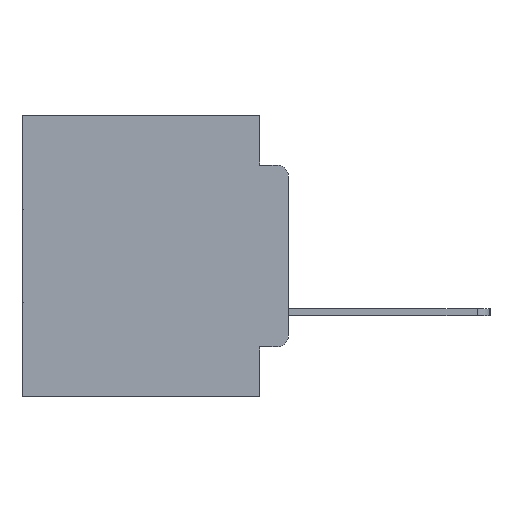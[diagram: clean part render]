
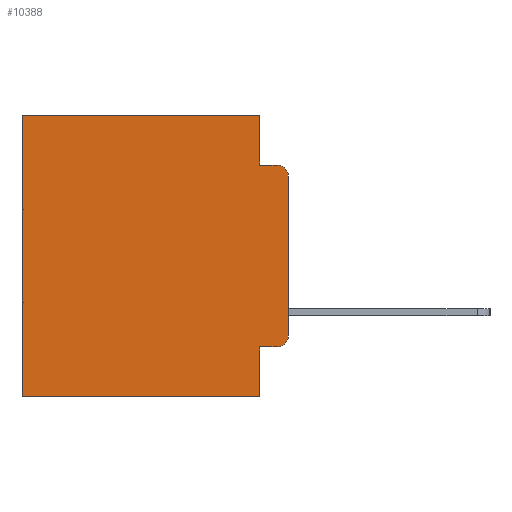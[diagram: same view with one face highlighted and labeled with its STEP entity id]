
A CAD part, left-side view. The second image highlights one B-rep face of the part: STEP entity #10388.
In plain terms, the highlighted planar face has unit normal (-1, 0, 0).
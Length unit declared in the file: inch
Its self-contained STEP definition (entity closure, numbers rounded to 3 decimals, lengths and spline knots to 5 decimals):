
#510 = ORIENTED_EDGE ( 'NONE', *, *, #28568, .F. ) ;
#564 = VECTOR ( 'NONE', #5904, 39.37008 ) ;
#1203 = ORIENTED_EDGE ( 'NONE', *, *, #3495, .T. ) ;
#1322 = AXIS2_PLACEMENT_3D ( 'NONE', #4643, #14088, #23806 ) ;
#1446 = CARTESIAN_POINT ( 'NONE',  ( 0.298, 0.02, -0.3915 ) ) ;
#1926 = DIRECTION ( 'NONE',  ( 0., 1., 0. ) ) ;
#1965 = LINE ( 'NONE', #17037, #8187 ) ;
#2395 = EDGE_CURVE ( 'NONE', #29765, #22675, #1965, .T. ) ;
#2718 = ORIENTED_EDGE ( 'NONE', *, *, #6503, .F. ) ;
#3455 = VERTEX_POINT ( 'NONE', #12804 ) ;
#3495 = EDGE_CURVE ( 'NONE', #3455, #20272, #7754, .T. ) ;
#3798 = DIRECTION ( 'NONE',  ( -1., 0., 0. ) ) ;
#4092 = CARTESIAN_POINT ( 'NONE',  ( 0.298, 0.051, -0.0885 ) ) ;
#4596 = EDGE_CURVE ( 'NONE', #22675, #9555, #8041, .T. ) ;
#4643 = CARTESIAN_POINT ( 'NONE',  ( 0.298, 0., 0. ) ) ;
#5254 = DIRECTION ( 'NONE',  ( 0., -1., 0. ) ) ;
#5904 = DIRECTION ( 'NONE',  ( 0., 0., -1. ) ) ;
#6090 = CARTESIAN_POINT ( 'NONE',  ( 0.298, 0.02, -0.0885 ) ) ;
#6092 = CARTESIAN_POINT ( 'NONE',  ( 0.298, 0., 0. ) ) ;
#6503 = EDGE_CURVE ( 'NONE', #11661, #7931, #19346, .T. ) ;
#6754 = VERTEX_POINT ( 'NONE', #18644 ) ;
#7508 = ORIENTED_EDGE ( 'NONE', *, *, #7940, .T. ) ;
#7754 = CIRCLE ( 'NONE', #28456, 0.02 ) ;
#7821 = VECTOR ( 'NONE', #1926, 39.37008 ) ;
#7931 = VERTEX_POINT ( 'NONE', #16019 ) ;
#7940 = EDGE_CURVE ( 'NONE', #29765, #28652, #14872, .T. ) ;
#7986 = VECTOR ( 'NONE', #17006, 39.37008 ) ;
#8041 = LINE ( 'NONE', #11181, #13588 ) ;
#8187 = VECTOR ( 'NONE', #28602, 39.37008 ) ;
#8257 = CARTESIAN_POINT ( 'NONE',  ( 0.298, 0.051, 0. ) ) ;
#8889 = EDGE_CURVE ( 'NONE', #6754, #9555, #11824, .T. ) ;
#9555 = VERTEX_POINT ( 'NONE', #6090 ) ;
#9933 = VECTOR ( 'NONE', #5254, 39.37008 ) ;
#10388 = ADVANCED_FACE ( 'NONE', ( #26729 ), #21034, .F. ) ;
#11032 = CARTESIAN_POINT ( 'NONE',  ( 0.298, 0.473, 0. ) ) ;
#11181 = CARTESIAN_POINT ( 'NONE',  ( 0.298, 0.051, -0.0885 ) ) ;
#11661 = VERTEX_POINT ( 'NONE', #22491 ) ;
#11824 = CIRCLE ( 'NONE', #20579, 0.02 ) ;
#12804 = CARTESIAN_POINT ( 'NONE',  ( 0.298, 0.02, -0.4115 ) ) ;
#13052 = ORIENTED_EDGE ( 'NONE', *, *, #4596, .F. ) ;
#13211 = ORIENTED_EDGE ( 'NONE', *, *, #14750, .T. ) ;
#13511 = ORIENTED_EDGE ( 'NONE', *, *, #8889, .T. ) ;
#13588 = VECTOR ( 'NONE', #24161, 39.37008 ) ;
#14088 = DIRECTION ( 'NONE',  ( 1., 0., 0. ) ) ;
#14274 = LINE ( 'NONE', #14643, #7986 ) ;
#14643 = CARTESIAN_POINT ( 'NONE',  ( 0.298, 0., -0.5 ) ) ;
#14750 = EDGE_CURVE ( 'NONE', #28652, #25594, #19076, .T. ) ;
#14872 = LINE ( 'NONE', #23047, #7821 ) ;
#15277 = ORIENTED_EDGE ( 'NONE', *, *, #2395, .F. ) ;
#16019 = CARTESIAN_POINT ( 'NONE',  ( 0.298, 0.051, -0.5 ) ) ;
#16219 = LINE ( 'NONE', #28557, #9933 ) ;
#16280 = CARTESIAN_POINT ( 'NONE',  ( 0.298, 0., -0.3915 ) ) ;
#16448 = EDGE_CURVE ( 'NONE', #6754, #20272, #23694, .T. ) ;
#16746 = ORIENTED_EDGE ( 'NONE', *, *, #16448, .F. ) ;
#17006 = DIRECTION ( 'NONE',  ( 0., 1., 0. ) ) ;
#17037 = CARTESIAN_POINT ( 'NONE',  ( 0.298, 0.051, 0. ) ) ;
#17871 = CARTESIAN_POINT ( 'NONE',  ( 0.298, 0.02, -0.1085 ) ) ;
#18644 = CARTESIAN_POINT ( 'NONE',  ( 0.298, 0., -0.1085 ) ) ;
#19076 = LINE ( 'NONE', #11032, #29229 ) ;
#19346 = LINE ( 'NONE', #8257, #564 ) ;
#20206 = DIRECTION ( 'NONE',  ( 0., 0., -1. ) ) ;
#20272 = VERTEX_POINT ( 'NONE', #16280 ) ;
#20465 = DIRECTION ( 'NONE',  ( 0., 0., -1. ) ) ;
#20579 = AXIS2_PLACEMENT_3D ( 'NONE', #17871, #3798, #20206 ) ;
#20928 = CARTESIAN_POINT ( 'NONE',  ( 0.298, 0.473, -0.5 ) ) ;
#21034 = PLANE ( 'NONE',  #1322 ) ;
#21976 = CARTESIAN_POINT ( 'NONE',  ( 0.298, 0.473, 0. ) ) ;
#22491 = CARTESIAN_POINT ( 'NONE',  ( 0.298, 0.051, -0.4115 ) ) ;
#22675 = VERTEX_POINT ( 'NONE', #4092 ) ;
#22955 = VECTOR ( 'NONE', #27169, 39.37008 ) ;
#23047 = CARTESIAN_POINT ( 'NONE',  ( 0.298, 0., 0. ) ) ;
#23694 = LINE ( 'NONE', #6092, #22955 ) ;
#23806 = DIRECTION ( 'NONE',  ( 0., 0., -1. ) ) ;
#23841 = EDGE_LOOP ( 'NONE', ( #16746, #13511, #13052, #15277, #7508, #13211, #510, #2718, #25213, #1203 ) ) ;
#23843 = CARTESIAN_POINT ( 'NONE',  ( 0.298, 0.051, 0. ) ) ;
#24161 = DIRECTION ( 'NONE',  ( 0., -1., 0. ) ) ;
#24799 = DIRECTION ( 'NONE',  ( 0., 0., -1. ) ) ;
#25213 = ORIENTED_EDGE ( 'NONE', *, *, #27016, .T. ) ;
#25227 = DIRECTION ( 'NONE',  ( -1., 0., 0. ) ) ;
#25594 = VERTEX_POINT ( 'NONE', #20928 ) ;
#26729 = FACE_OUTER_BOUND ( 'NONE', #23841, .T. ) ;
#27016 = EDGE_CURVE ( 'NONE', #11661, #3455, #16219, .T. ) ;
#27169 = DIRECTION ( 'NONE',  ( 0., 0., -1. ) ) ;
#28456 = AXIS2_PLACEMENT_3D ( 'NONE', #1446, #25227, #24799 ) ;
#28557 = CARTESIAN_POINT ( 'NONE',  ( 0.298, 0.051, -0.4115 ) ) ;
#28568 = EDGE_CURVE ( 'NONE', #7931, #25594, #14274, .T. ) ;
#28602 = DIRECTION ( 'NONE',  ( 0., 0., -1. ) ) ;
#28652 = VERTEX_POINT ( 'NONE', #21976 ) ;
#29229 = VECTOR ( 'NONE', #20465, 39.37008 ) ;
#29765 = VERTEX_POINT ( 'NONE', #23843 ) ;
